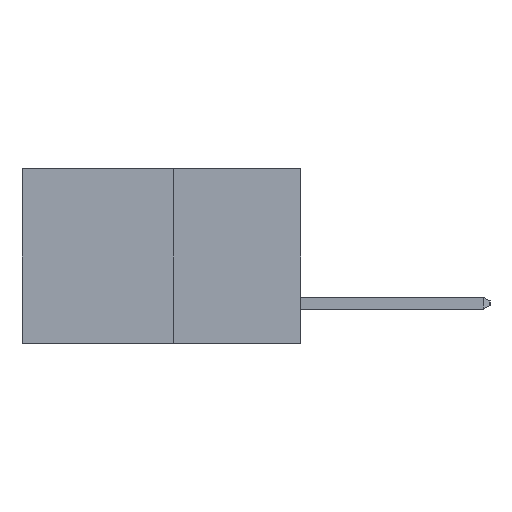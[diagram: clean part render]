
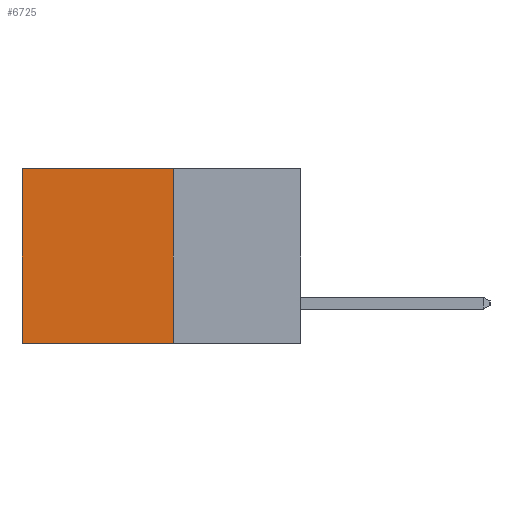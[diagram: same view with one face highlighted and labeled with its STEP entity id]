
A CAD part, left-side view. The second image highlights one B-rep face of the part: STEP entity #6725.
In plain terms, the highlighted planar face has unit normal (-1, 0, 0).
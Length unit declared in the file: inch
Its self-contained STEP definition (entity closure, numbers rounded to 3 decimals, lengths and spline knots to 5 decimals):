
#233 = CARTESIAN_POINT ( 'NONE',  ( 0.277, 0.59, -0.37 ) ) ;
#380 = ORIENTED_EDGE ( 'NONE', *, *, #7134, .T. ) ;
#472 = VERTEX_POINT ( 'NONE', #3272 ) ;
#1162 = CARTESIAN_POINT ( 'NONE',  ( 0.277, 0.27, -0.37 ) ) ;
#1402 = EDGE_CURVE ( 'NONE', #2126, #6670, #3816, .T. ) ;
#1490 = DIRECTION ( 'NONE',  ( 0., 0., -1. ) ) ;
#2106 = EDGE_CURVE ( 'NONE', #472, #2126, #3527, .T. ) ;
#2126 = VERTEX_POINT ( 'NONE', #8812 ) ;
#2194 = ORIENTED_EDGE ( 'NONE', *, *, #4198, .T. ) ;
#2416 = DIRECTION ( 'NONE',  ( 0., 0., -1. ) ) ;
#2567 = AXIS2_PLACEMENT_3D ( 'NONE', #8334, #5640, #1490 ) ;
#2802 = DIRECTION ( 'NONE',  ( 0., 0., -1. ) ) ;
#2928 = LINE ( 'NONE', #7266, #6338 ) ;
#3192 = DIRECTION ( 'NONE',  ( 0., 1., 0. ) ) ;
#3272 = CARTESIAN_POINT ( 'NONE',  ( 0.277, 0.27, 0. ) ) ;
#3300 = VECTOR ( 'NONE', #2802, 39.37008 ) ;
#3527 = LINE ( 'NONE', #1162, #3300 ) ;
#3658 = VERTEX_POINT ( 'NONE', #4969 ) ;
#3816 = LINE ( 'NONE', #3984, #7194 ) ;
#3984 = CARTESIAN_POINT ( 'NONE',  ( 0.277, 0.27, -0.37 ) ) ;
#4198 = EDGE_CURVE ( 'NONE', #3658, #6670, #6556, .T. ) ;
#4389 = ORIENTED_EDGE ( 'NONE', *, *, #2106, .F. ) ;
#4866 = EDGE_LOOP ( 'NONE', ( #2194, #6894, #4389, #380 ) ) ;
#4969 = CARTESIAN_POINT ( 'NONE',  ( 0.277, 0.59, 0. ) ) ;
#5608 = PLANE ( 'NONE',  #2567 ) ;
#5640 = DIRECTION ( 'NONE',  ( 1., 0., 0. ) ) ;
#5663 = DIRECTION ( 'NONE',  ( 0., 1., 0. ) ) ;
#6338 = VECTOR ( 'NONE', #3192, 39.37008 ) ;
#6556 = LINE ( 'NONE', #233, #8556 ) ;
#6670 = VERTEX_POINT ( 'NONE', #7612 ) ;
#6725 = ADVANCED_FACE ( 'NONE', ( #8172 ), #5608, .F. ) ;
#6894 = ORIENTED_EDGE ( 'NONE', *, *, #1402, .F. ) ;
#7134 = EDGE_CURVE ( 'NONE', #472, #3658, #2928, .T. ) ;
#7194 = VECTOR ( 'NONE', #5663, 39.37008 ) ;
#7266 = CARTESIAN_POINT ( 'NONE',  ( 0.277, 0.27, 0. ) ) ;
#7612 = CARTESIAN_POINT ( 'NONE',  ( 0.277, 0.59, -0.37 ) ) ;
#8172 = FACE_OUTER_BOUND ( 'NONE', #4866, .T. ) ;
#8334 = CARTESIAN_POINT ( 'NONE',  ( 0.277, 0.27, -0.37 ) ) ;
#8556 = VECTOR ( 'NONE', #2416, 39.37008 ) ;
#8812 = CARTESIAN_POINT ( 'NONE',  ( 0.277, 0.27, -0.37 ) ) ;
